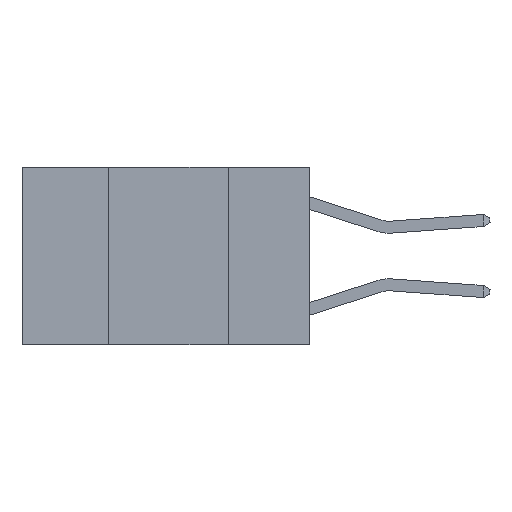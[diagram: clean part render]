
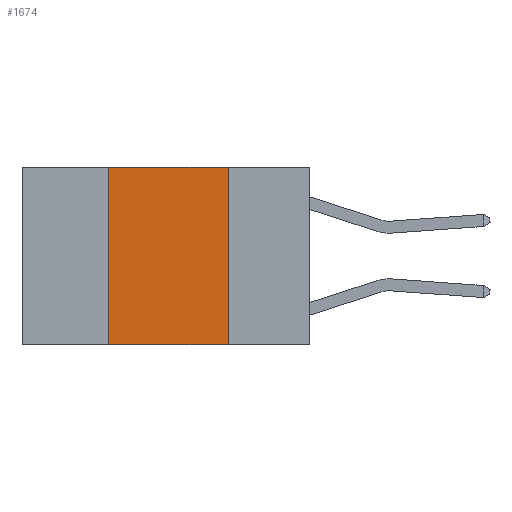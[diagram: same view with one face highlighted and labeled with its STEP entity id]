
A CAD part, left-side view. The second image highlights one B-rep face of the part: STEP entity #1674.
In plain terms, the highlighted planar face has unit normal (-1, 0, 0).
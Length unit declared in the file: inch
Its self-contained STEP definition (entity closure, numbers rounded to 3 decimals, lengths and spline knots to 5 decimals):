
#401 = EDGE_LOOP ( 'NONE', ( #6723, #812, #861, #4930 ) ) ;
#668 = PLANE ( 'NONE',  #2559 ) ;
#812 = ORIENTED_EDGE ( 'NONE', *, *, #8765, .F. ) ;
#861 = ORIENTED_EDGE ( 'NONE', *, *, #885, .F. ) ;
#885 = EDGE_CURVE ( 'NONE', #7422, #11501, #12744, .T. ) ;
#1043 = CARTESIAN_POINT ( 'NONE',  ( 0., 0.42, -0.37 ) ) ;
#1674 = ADVANCED_FACE ( 'NONE', ( #12881 ), #668, .F. ) ;
#1729 = CARTESIAN_POINT ( 'NONE',  ( 0., 0.6, 0. ) ) ;
#1998 = VECTOR ( 'NONE', #9175, 39.37008 ) ;
#2021 = CARTESIAN_POINT ( 'NONE',  ( 0., 0.17, 0. ) ) ;
#2290 = VERTEX_POINT ( 'NONE', #2021 ) ;
#2559 = AXIS2_PLACEMENT_3D ( 'NONE', #12808, #2796, #11823 ) ;
#2796 = DIRECTION ( 'NONE',  ( 1., 0., 0. ) ) ;
#2868 = DIRECTION ( 'NONE',  ( 0., -1., 0. ) ) ;
#3436 = VERTEX_POINT ( 'NONE', #9930 ) ;
#4511 = DIRECTION ( 'NONE',  ( 0., 0., 1. ) ) ;
#4568 = LINE ( 'NONE', #1729, #11680 ) ;
#4930 = ORIENTED_EDGE ( 'NONE', *, *, #6078, .T. ) ;
#5556 = CARTESIAN_POINT ( 'NONE',  ( 0., 0.42, 0. ) ) ;
#5923 = CARTESIAN_POINT ( 'NONE',  ( 0., 0.6, -0.37 ) ) ;
#6078 = EDGE_CURVE ( 'NONE', #7422, #3436, #11867, .T. ) ;
#6107 = DIRECTION ( 'NONE',  ( 0., -1., 0. ) ) ;
#6723 = ORIENTED_EDGE ( 'NONE', *, *, #9755, .F. ) ;
#6964 = LINE ( 'NONE', #9100, #1998 ) ;
#7422 = VERTEX_POINT ( 'NONE', #1043 ) ;
#8765 = EDGE_CURVE ( 'NONE', #11501, #2290, #4568, .T. ) ;
#9100 = CARTESIAN_POINT ( 'NONE',  ( 0., 0.17, 0. ) ) ;
#9175 = DIRECTION ( 'NONE',  ( 0., 0., -1. ) ) ;
#9755 = EDGE_CURVE ( 'NONE', #2290, #3436, #6964, .T. ) ;
#9930 = CARTESIAN_POINT ( 'NONE',  ( 0., 0.17, -0.37 ) ) ;
#11121 = VECTOR ( 'NONE', #4511, 39.37008 ) ;
#11501 = VERTEX_POINT ( 'NONE', #12008 ) ;
#11680 = VECTOR ( 'NONE', #2868, 39.37008 ) ;
#11823 = DIRECTION ( 'NONE',  ( 0., 0., -1. ) ) ;
#11852 = VECTOR ( 'NONE', #6107, 39.37008 ) ;
#11867 = LINE ( 'NONE', #5923, #11852 ) ;
#12008 = CARTESIAN_POINT ( 'NONE',  ( 0., 0.42, 0. ) ) ;
#12744 = LINE ( 'NONE', #5556, #11121 ) ;
#12808 = CARTESIAN_POINT ( 'NONE',  ( 0., 0.6, 0. ) ) ;
#12881 = FACE_OUTER_BOUND ( 'NONE', #401, .T. ) ;
